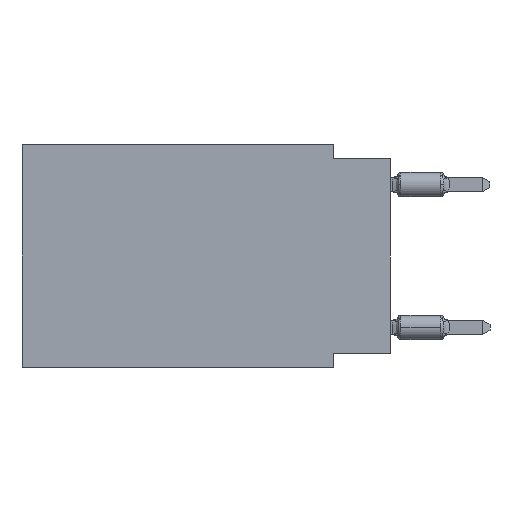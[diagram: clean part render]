
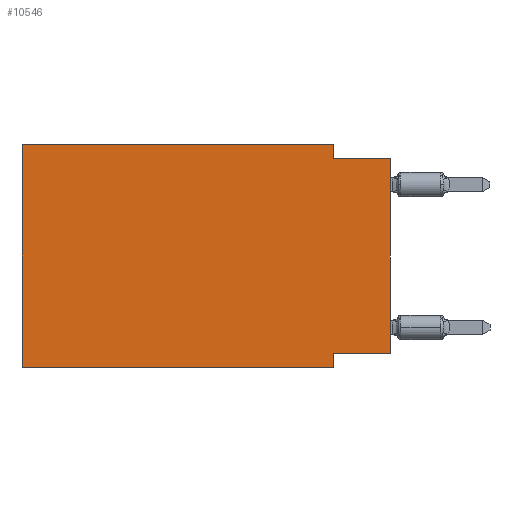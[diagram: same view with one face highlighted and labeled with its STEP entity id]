
A CAD part, left-side view. The second image highlights one B-rep face of the part: STEP entity #10546.
In plain terms, the highlighted planar face has unit normal (-1, 0, 0).
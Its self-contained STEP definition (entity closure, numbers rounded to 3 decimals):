
#183 = CARTESIAN_POINT ( 'NONE',  ( 0., 16.383, 0. ) ) ;
#205 = LINE ( 'NONE', #11781, #9643 ) ;
#465 = LINE ( 'NONE', #3279, #18409 ) ;
#861 = ORIENTED_EDGE ( 'NONE', *, *, #11814, .F. ) ;
#915 = CARTESIAN_POINT ( 'NONE',  ( 0., 16.383, 0. ) ) ;
#1550 = AXIS2_PLACEMENT_3D ( 'NONE', #183, #8731, #10432 ) ;
#1553 = LINE ( 'NONE', #3150, #1569 ) ;
#1569 = VECTOR ( 'NONE', #3053, 1000. ) ;
#1590 = FACE_OUTER_BOUND ( 'NONE', #18036, .T. ) ;
#2003 = VERTEX_POINT ( 'NONE', #915 ) ;
#2878 = EDGE_CURVE ( 'NONE', #6206, #17498, #6795, .T. ) ;
#2935 = EDGE_CURVE ( 'NONE', #10312, #13468, #465, .T. ) ;
#3053 = DIRECTION ( 'NONE',  ( 0., -1., 0. ) ) ;
#3150 = CARTESIAN_POINT ( 'NONE',  ( 0., 0., -0.635 ) ) ;
#3279 = CARTESIAN_POINT ( 'NONE',  ( 0., 0., -9.271 ) ) ;
#3950 = VECTOR ( 'NONE', #10704, 1000. ) ;
#5116 = ORIENTED_EDGE ( 'NONE', *, *, #2935, .F. ) ;
#5384 = DIRECTION ( 'NONE',  ( 0., 0., -1. ) ) ;
#5957 = EDGE_CURVE ( 'NONE', #11267, #2003, #9323, .T. ) ;
#6089 = CARTESIAN_POINT ( 'NONE',  ( 0., 0., -0.635 ) ) ;
#6206 = VERTEX_POINT ( 'NONE', #7254 ) ;
#6385 = CARTESIAN_POINT ( 'NONE',  ( 0., 0., -9.271 ) ) ;
#6501 = EDGE_CURVE ( 'NONE', #11267, #17703, #16809, .T. ) ;
#6795 = LINE ( 'NONE', #12537, #9121 ) ;
#7005 = ORIENTED_EDGE ( 'NONE', *, *, #7890, .F. ) ;
#7103 = VECTOR ( 'NONE', #11892, 1000. ) ;
#7254 = CARTESIAN_POINT ( 'NONE',  ( 0., 2.54, 0. ) ) ;
#7327 = PLANE ( 'NONE',  #1550 ) ;
#7377 = CARTESIAN_POINT ( 'NONE',  ( 0., 2.54, -0.635 ) ) ;
#7421 = CARTESIAN_POINT ( 'NONE',  ( 0., 0., 0. ) ) ;
#7608 = DIRECTION ( 'NONE',  ( 0., 1., 0. ) ) ;
#7890 = EDGE_CURVE ( 'NONE', #2003, #6206, #14446, .T. ) ;
#7905 = CARTESIAN_POINT ( 'NONE',  ( 0., 16.383, 0. ) ) ;
#7986 = VECTOR ( 'NONE', #13815, 1000. ) ;
#8731 = DIRECTION ( 'NONE',  ( 1., 0., 0. ) ) ;
#9106 = LINE ( 'NONE', #7421, #3950 ) ;
#9121 = VECTOR ( 'NONE', #5384, 1000. ) ;
#9323 = LINE ( 'NONE', #7905, #7103 ) ;
#9643 = VECTOR ( 'NONE', #17497, 1000. ) ;
#9933 = DIRECTION ( 'NONE',  ( 0., -1., 0. ) ) ;
#10200 = EDGE_CURVE ( 'NONE', #13468, #17703, #205, .T. ) ;
#10312 = VERTEX_POINT ( 'NONE', #6385 ) ;
#10432 = DIRECTION ( 'NONE',  ( 0., 0., -1. ) ) ;
#10546 = ADVANCED_FACE ( 'NONE', ( #1590 ), #7327, .F. ) ;
#10578 = EDGE_CURVE ( 'NONE', #10312, #15452, #9106, .T. ) ;
#10704 = DIRECTION ( 'NONE',  ( 0., 0., 1. ) ) ;
#11267 = VERTEX_POINT ( 'NONE', #16096 ) ;
#11781 = CARTESIAN_POINT ( 'NONE',  ( 0., 2.54, -9.906 ) ) ;
#11814 = EDGE_CURVE ( 'NONE', #17498, #15452, #1553, .T. ) ;
#11834 = ORIENTED_EDGE ( 'NONE', *, *, #2878, .F. ) ;
#11892 = DIRECTION ( 'NONE',  ( 0., 0., 1. ) ) ;
#12265 = ORIENTED_EDGE ( 'NONE', *, *, #6501, .T. ) ;
#12537 = CARTESIAN_POINT ( 'NONE',  ( 0., 2.54, 0. ) ) ;
#13416 = ORIENTED_EDGE ( 'NONE', *, *, #10200, .F. ) ;
#13468 = VERTEX_POINT ( 'NONE', #15460 ) ;
#13815 = DIRECTION ( 'NONE',  ( 0., -1., 0. ) ) ;
#14047 = ORIENTED_EDGE ( 'NONE', *, *, #10578, .T. ) ;
#14446 = LINE ( 'NONE', #15938, #15459 ) ;
#15452 = VERTEX_POINT ( 'NONE', #6089 ) ;
#15459 = VECTOR ( 'NONE', #9933, 1000. ) ;
#15460 = CARTESIAN_POINT ( 'NONE',  ( 0., 2.54, -9.271 ) ) ;
#15938 = CARTESIAN_POINT ( 'NONE',  ( 0., 16.383, 0. ) ) ;
#16096 = CARTESIAN_POINT ( 'NONE',  ( 0., 16.383, -9.906 ) ) ;
#16350 = ORIENTED_EDGE ( 'NONE', *, *, #5957, .F. ) ;
#16558 = CARTESIAN_POINT ( 'NONE',  ( 0., 2.54, -9.906 ) ) ;
#16809 = LINE ( 'NONE', #18031, #7986 ) ;
#17497 = DIRECTION ( 'NONE',  ( 0., 0., -1. ) ) ;
#17498 = VERTEX_POINT ( 'NONE', #7377 ) ;
#17703 = VERTEX_POINT ( 'NONE', #16558 ) ;
#18031 = CARTESIAN_POINT ( 'NONE',  ( 0., 16.383, -9.906 ) ) ;
#18036 = EDGE_LOOP ( 'NONE', ( #14047, #861, #11834, #7005, #16350, #12265, #13416, #5116 ) ) ;
#18409 = VECTOR ( 'NONE', #7608, 1000. ) ;
